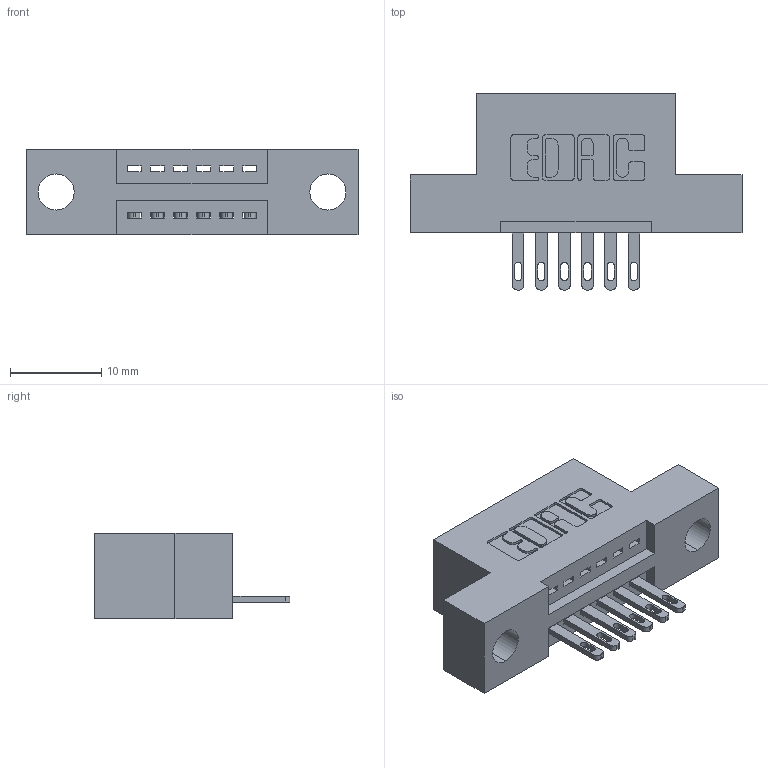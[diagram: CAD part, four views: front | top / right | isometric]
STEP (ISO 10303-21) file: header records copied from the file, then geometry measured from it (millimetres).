
FILE_DESCRIPTION (( 'STEP AP203' ), '1' );
FILE_NAME ('345-006-500-104.STEP', '2018-08-16T22:53:49', ( '' ), ( '' ), 'SwSTEP 2.0', 'SolidWorks 2016', '' );
FILE_SCHEMA (( 'CONFIG_CONTROL_DESIGN' ));
Length unit declared in the file: inch
Products named in the file (3): 345 Part_Flush Mounting Lugs - 0.156 Dia-TH; 345-292-001_345-293-100; 345-006-500-104
Assembly tree (7 placements, depth 2):
  345-006-500-104
    345 Part_Flush Mounting Lugs - 0.156 Dia-TH
    345-292-001_345-293-100  x6
Bounding box: 36.45 x 21.51 x 9.4 mm (x, y, z)
Volume: 3082.9 mm3; surface area: 3429.9 mm2
Topology: 7 solids, 7 shells, 450 faces, 1349 edges, 898 vertices
Faces by surface type: plane 284, cylinder 166
Entity records: 9295 total; most frequent: CARTESIAN_POINT 1618, ORIENTED_EDGE 1558, DIRECTION 1467, EDGE_CURVE 779, VECTOR 619, LINE 619, VERTEX_POINT 518, AXIS2_PLACEMENT_3D 424
